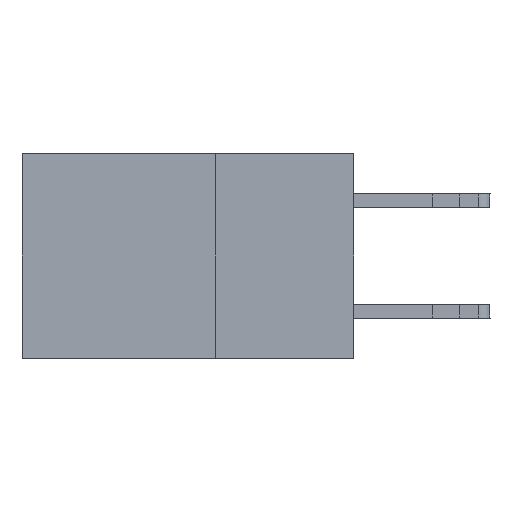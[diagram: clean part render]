
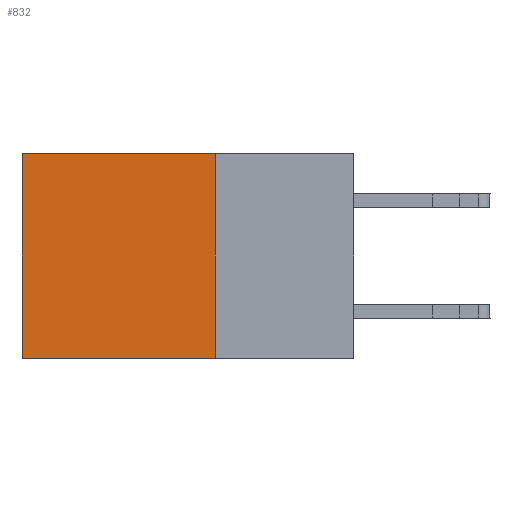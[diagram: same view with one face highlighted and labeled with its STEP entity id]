
A CAD part, left-side view. The second image highlights one B-rep face of the part: STEP entity #832.
In plain terms, the highlighted planar face has unit normal (-1, 0, 0).
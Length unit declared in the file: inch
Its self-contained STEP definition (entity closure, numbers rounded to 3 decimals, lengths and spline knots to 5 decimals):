
#832 = ADVANCED_FACE ( 'NONE', ( #17617 ), #4354, .F. ) ;
#1003 = VECTOR ( 'NONE', #32394, 39.37008 ) ;
#1057 = ORIENTED_EDGE ( 'NONE', *, *, #12493, .T. ) ;
#1768 = CARTESIAN_POINT ( 'NONE',  ( 0.2875, 0.25, 0. ) ) ;
#2102 = VERTEX_POINT ( 'NONE', #14058 ) ;
#2172 = EDGE_CURVE ( 'NONE', #27959, #27228, #30020, .T. ) ;
#3580 = CARTESIAN_POINT ( 'NONE',  ( 0.2875, 0.25, 0. ) ) ;
#4354 = PLANE ( 'NONE',  #26914 ) ;
#4524 = DIRECTION ( 'NONE',  ( 0., 0., -1. ) ) ;
#5400 = CARTESIAN_POINT ( 'NONE',  ( 0.2875, 0.6, 0. ) ) ;
#6216 = VECTOR ( 'NONE', #11303, 39.37008 ) ;
#7384 = CARTESIAN_POINT ( 'NONE',  ( 0.2875, 0.25, -0.37 ) ) ;
#8910 = DIRECTION ( 'NONE',  ( 0., 0., -1. ) ) ;
#8993 = VERTEX_POINT ( 'NONE', #7384 ) ;
#9402 = DIRECTION ( 'NONE',  ( 0., 0., -1. ) ) ;
#9803 = VECTOR ( 'NONE', #8910, 39.37008 ) ;
#9907 = LINE ( 'NONE', #3580, #9803 ) ;
#10911 = CARTESIAN_POINT ( 'NONE',  ( 0.2875, 0.25, -0.37 ) ) ;
#11303 = DIRECTION ( 'NONE',  ( 0., 1., 0. ) ) ;
#11432 = EDGE_CURVE ( 'NONE', #8993, #2102, #16751, .T. ) ;
#12493 = EDGE_CURVE ( 'NONE', #27228, #2102, #17143, .T. ) ;
#13316 = ORIENTED_EDGE ( 'NONE', *, *, #2172, .T. ) ;
#14058 = CARTESIAN_POINT ( 'NONE',  ( 0.2875, 0.6, -0.37 ) ) ;
#15557 = EDGE_CURVE ( 'NONE', #27959, #8993, #9907, .T. ) ;
#16751 = LINE ( 'NONE', #10911, #1003 ) ;
#16922 = DIRECTION ( 'NONE',  ( 1., 0., 0. ) ) ;
#17143 = LINE ( 'NONE', #22470, #21926 ) ;
#17617 = FACE_OUTER_BOUND ( 'NONE', #18404, .T. ) ;
#18404 = EDGE_LOOP ( 'NONE', ( #1057, #18495, #19011, #13316 ) ) ;
#18495 = ORIENTED_EDGE ( 'NONE', *, *, #11432, .F. ) ;
#19011 = ORIENTED_EDGE ( 'NONE', *, *, #15557, .F. ) ;
#21926 = VECTOR ( 'NONE', #9402, 39.37008 ) ;
#22470 = CARTESIAN_POINT ( 'NONE',  ( 0.2875, 0.6, 0. ) ) ;
#26914 = AXIS2_PLACEMENT_3D ( 'NONE', #1768, #16922, #4524 ) ;
#27228 = VERTEX_POINT ( 'NONE', #5400 ) ;
#27959 = VERTEX_POINT ( 'NONE', #33326 ) ;
#30020 = LINE ( 'NONE', #32787, #6216 ) ;
#32394 = DIRECTION ( 'NONE',  ( 0., 1., 0. ) ) ;
#32787 = CARTESIAN_POINT ( 'NONE',  ( 0.2875, 0.25, 0. ) ) ;
#33326 = CARTESIAN_POINT ( 'NONE',  ( 0.2875, 0.25, 0. ) ) ;
